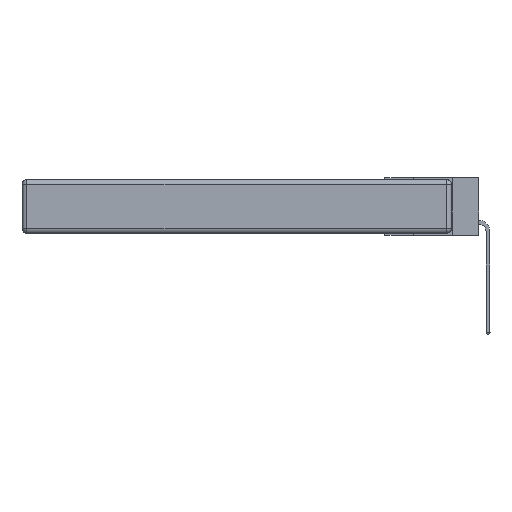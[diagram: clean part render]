
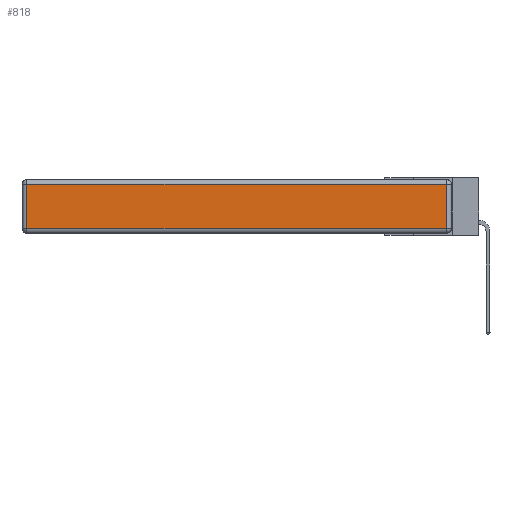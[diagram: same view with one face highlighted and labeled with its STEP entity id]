
A CAD part, left-side view. The second image highlights one B-rep face of the part: STEP entity #818.
In plain terms, the highlighted planar face has unit normal (-1, 0, 0).
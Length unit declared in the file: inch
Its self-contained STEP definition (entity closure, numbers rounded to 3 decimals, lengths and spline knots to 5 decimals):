
#818 = ADVANCED_FACE ( 'NONE', ( #3735 ), #18195, .T. ) ;
#1221 = VECTOR ( 'NONE', #20609, 39.37008 ) ;
#1409 = VERTEX_POINT ( 'NONE', #20323 ) ;
#1507 = VECTOR ( 'NONE', #21194, 39.37008 ) ;
#1885 = DIRECTION ( 'NONE',  ( 0., -1., 0. ) ) ;
#2682 = LINE ( 'NONE', #19380, #1507 ) ;
#2868 = EDGE_LOOP ( 'NONE', ( #18497, #16426, #4058, #8259 ) ) ;
#3512 = LINE ( 'NONE', #16790, #19164 ) ;
#3735 = FACE_OUTER_BOUND ( 'NONE', #2868, .T. ) ;
#4058 = ORIENTED_EDGE ( 'NONE', *, *, #9402, .T. ) ;
#7129 = DIRECTION ( 'NONE',  ( -1., 0., 0. ) ) ;
#7221 = CARTESIAN_POINT ( 'NONE',  ( 0., 2.72, -0.343 ) ) ;
#8202 = EDGE_CURVE ( 'NONE', #23387, #19898, #2682, .T. ) ;
#8259 = ORIENTED_EDGE ( 'NONE', *, *, #14076, .T. ) ;
#9402 = EDGE_CURVE ( 'NONE', #19898, #1409, #9956, .T. ) ;
#9956 = LINE ( 'NONE', #11504, #10520 ) ;
#10520 = VECTOR ( 'NONE', #13229, 39.37008 ) ;
#11223 = LINE ( 'NONE', #7221, #1221 ) ;
#11504 = CARTESIAN_POINT ( 'NONE',  ( 0., 2.75, -0.03 ) ) ;
#12659 = CARTESIAN_POINT ( 'NONE',  ( 0., 0., -0.343 ) ) ;
#13229 = DIRECTION ( 'NONE',  ( 0., 1., 0. ) ) ;
#14076 = EDGE_CURVE ( 'NONE', #1409, #16118, #11223, .T. ) ;
#16118 = VERTEX_POINT ( 'NONE', #21367 ) ;
#16426 = ORIENTED_EDGE ( 'NONE', *, *, #8202, .T. ) ;
#16777 = CARTESIAN_POINT ( 'NONE',  ( 0., 0.03, -0.313 ) ) ;
#16790 = CARTESIAN_POINT ( 'NONE',  ( 0., 0., -0.313 ) ) ;
#17830 = CARTESIAN_POINT ( 'NONE',  ( 0., 0.03, -0.03 ) ) ;
#18195 = PLANE ( 'NONE',  #18583 ) ;
#18497 = ORIENTED_EDGE ( 'NONE', *, *, #22159, .T. ) ;
#18583 = AXIS2_PLACEMENT_3D ( 'NONE', #12659, #7129, #20272 ) ;
#19164 = VECTOR ( 'NONE', #1885, 39.37008 ) ;
#19380 = CARTESIAN_POINT ( 'NONE',  ( 0., 0.03, -0.343 ) ) ;
#19898 = VERTEX_POINT ( 'NONE', #17830 ) ;
#20272 = DIRECTION ( 'NONE',  ( 0., 0., 1. ) ) ;
#20323 = CARTESIAN_POINT ( 'NONE',  ( 0., 2.72, -0.03 ) ) ;
#20609 = DIRECTION ( 'NONE',  ( 0., 0., -1. ) ) ;
#21194 = DIRECTION ( 'NONE',  ( 0., 0., 1. ) ) ;
#21367 = CARTESIAN_POINT ( 'NONE',  ( 0., 2.72, -0.313 ) ) ;
#22159 = EDGE_CURVE ( 'NONE', #16118, #23387, #3512, .T. ) ;
#23387 = VERTEX_POINT ( 'NONE', #16777 ) ;
